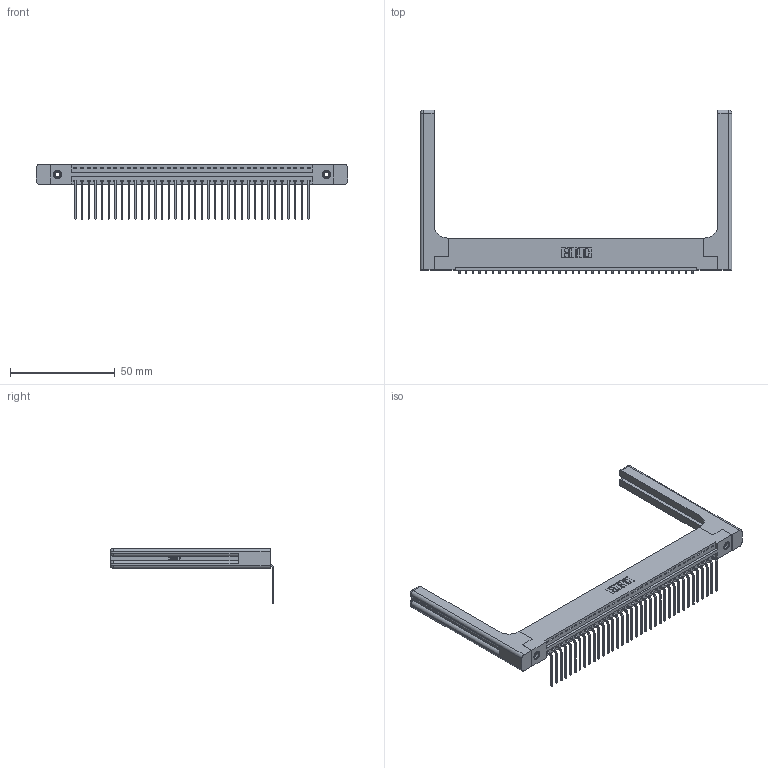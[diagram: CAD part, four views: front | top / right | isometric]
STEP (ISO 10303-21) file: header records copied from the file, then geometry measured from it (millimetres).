
FILE_DESCRIPTION (( 'STEP AP203' ), '1' );
FILE_NAME ('346-036-559-158.STEP', '2022-05-07T01:46:41', ( '' ), ( '' ), 'SwSTEP 2.0', 'SolidWorks 2020', '' );
FILE_SCHEMA (( 'CONFIG_CONTROL_DESIGN' ));
Length unit declared in the file: inch
Products named in the file (5): 345-250-001_345-250-001-102; 345-292-001_558 559 Tail - 1; 346 Part_Flush Mounting Lugs - 0.156 Dia-TH; 346-036-559-158; 346-220-058_345-220-058
Assembly tree (41 placements, depth 2):
  346-036-559-158
    346 Part_Flush Mounting Lugs - 0.156 Dia-TH
    345-292-001_558 559 Tail - 1  x36
    345-250-001_345-250-001-102  x2
    346-220-058_345-220-058  x2
Bounding box: 148.36 x 78.04 x 26.16 mm (x, y, z)
Volume: 21780.4 mm3; surface area: 23678.3 mm2
Topology: 41 solids, 41 shells, 2552 faces, 7583 edges, 4986 vertices
Faces by surface type: plane 1750, cylinder 742, bspline 36, cone 12, sphere 8, torus 4
Entity records: 28832 total; most frequent: CARTESIAN_POINT 5927, ORIENTED_EDGE 4692, DIRECTION 4166, EDGE_CURVE 2346, LINE 1978, VECTOR 1978, VERTEX_POINT 1554, AXIS2_PLACEMENT_3D 1094
